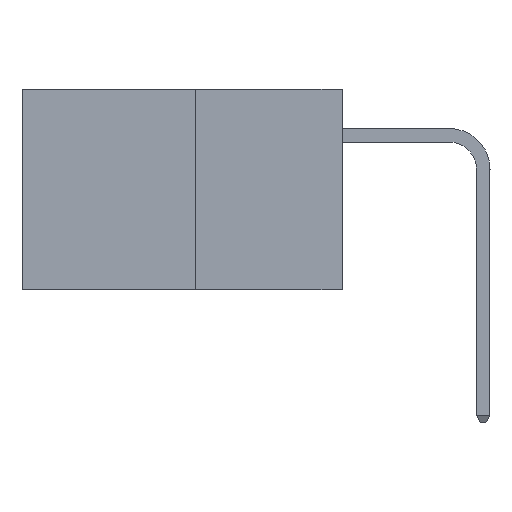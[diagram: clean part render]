
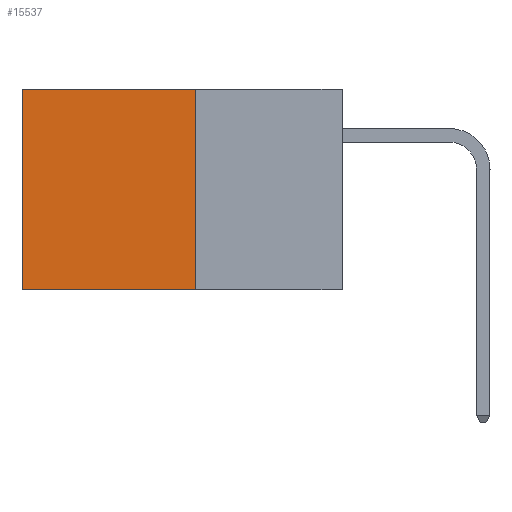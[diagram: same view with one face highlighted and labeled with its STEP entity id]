
A CAD part, left-side view. The second image highlights one B-rep face of the part: STEP entity #15537.
In plain terms, the highlighted planar face has unit normal (-1, 0, 0).
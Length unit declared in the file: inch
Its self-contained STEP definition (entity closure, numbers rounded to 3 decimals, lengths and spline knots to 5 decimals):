
#1265 = DIRECTION ( 'NONE',  ( 0., 1., 0. ) ) ;
#1388 = CARTESIAN_POINT ( 'NONE',  ( 0.277, 0.27, -0.37 ) ) ;
#3194 = CARTESIAN_POINT ( 'NONE',  ( 0.277, 0.59, 0. ) ) ;
#3508 = CARTESIAN_POINT ( 'NONE',  ( 0.277, 0.27, 0. ) ) ;
#3751 = LINE ( 'NONE', #20583, #18523 ) ;
#4035 = VECTOR ( 'NONE', #1265, 39.37008 ) ;
#5151 = CARTESIAN_POINT ( 'NONE',  ( 0.277, 0.27, -0.37 ) ) ;
#5724 = FACE_OUTER_BOUND ( 'NONE', #6213, .T. ) ;
#5873 = EDGE_CURVE ( 'NONE', #24275, #25618, #9522, .T. ) ;
#6105 = CARTESIAN_POINT ( 'NONE',  ( 0.277, 0.59, -0.37 ) ) ;
#6213 = EDGE_LOOP ( 'NONE', ( #25330, #19573, #16288, #18883 ) ) ;
#7872 = EDGE_CURVE ( 'NONE', #19344, #24275, #12592, .T. ) ;
#9306 = VECTOR ( 'NONE', #20052, 39.37008 ) ;
#9522 = LINE ( 'NONE', #1388, #4035 ) ;
#9975 = VERTEX_POINT ( 'NONE', #3194 ) ;
#11497 = CARTESIAN_POINT ( 'NONE',  ( 0.277, 0.27, -0.37 ) ) ;
#12266 = AXIS2_PLACEMENT_3D ( 'NONE', #11497, #25126, #13474 ) ;
#12592 = LINE ( 'NONE', #5151, #22432 ) ;
#13474 = DIRECTION ( 'NONE',  ( 0., 0., -1. ) ) ;
#15537 = ADVANCED_FACE ( 'NONE', ( #5724 ), #23221, .F. ) ;
#16288 = ORIENTED_EDGE ( 'NONE', *, *, #7872, .F. ) ;
#16709 = EDGE_CURVE ( 'NONE', #19344, #9975, #3751, .T. ) ;
#17304 = CARTESIAN_POINT ( 'NONE',  ( 0.277, 0.27, -0.37 ) ) ;
#18523 = VECTOR ( 'NONE', #20664, 39.37008 ) ;
#18883 = ORIENTED_EDGE ( 'NONE', *, *, #16709, .T. ) ;
#19171 = DIRECTION ( 'NONE',  ( 0., 0., -1. ) ) ;
#19224 = LINE ( 'NONE', #6105, #9306 ) ;
#19344 = VERTEX_POINT ( 'NONE', #3508 ) ;
#19573 = ORIENTED_EDGE ( 'NONE', *, *, #5873, .F. ) ;
#20052 = DIRECTION ( 'NONE',  ( 0., 0., -1. ) ) ;
#20583 = CARTESIAN_POINT ( 'NONE',  ( 0.277, 0.27, 0. ) ) ;
#20664 = DIRECTION ( 'NONE',  ( 0., 1., 0. ) ) ;
#20765 = EDGE_CURVE ( 'NONE', #9975, #25618, #19224, .T. ) ;
#21577 = CARTESIAN_POINT ( 'NONE',  ( 0.277, 0.59, -0.37 ) ) ;
#22432 = VECTOR ( 'NONE', #19171, 39.37008 ) ;
#23221 = PLANE ( 'NONE',  #12266 ) ;
#24275 = VERTEX_POINT ( 'NONE', #17304 ) ;
#25126 = DIRECTION ( 'NONE',  ( 1., 0., 0. ) ) ;
#25330 = ORIENTED_EDGE ( 'NONE', *, *, #20765, .T. ) ;
#25618 = VERTEX_POINT ( 'NONE', #21577 ) ;
